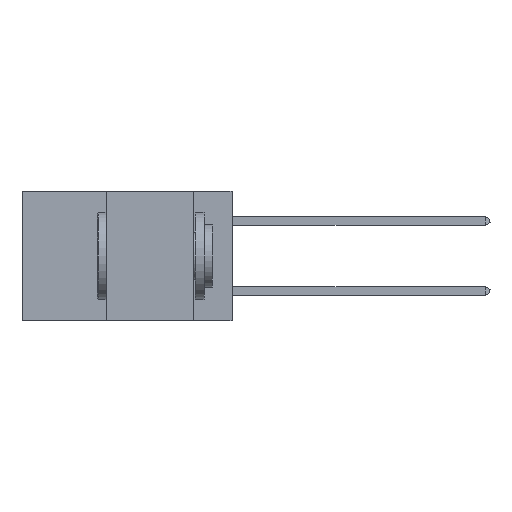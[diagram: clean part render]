
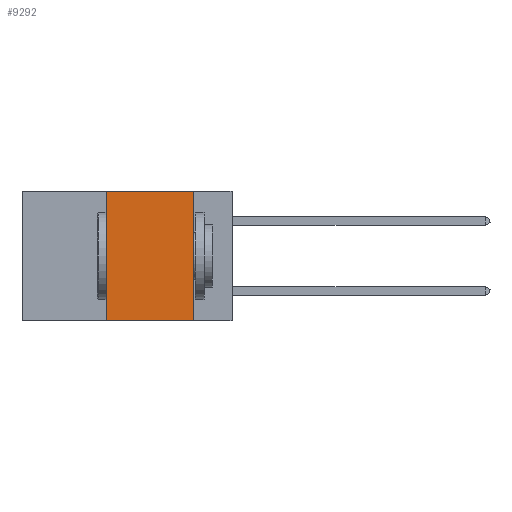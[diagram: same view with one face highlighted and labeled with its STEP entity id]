
A CAD part, left-side view. The second image highlights one B-rep face of the part: STEP entity #9292.
In plain terms, the highlighted planar face has unit normal (-1, 0, 0).
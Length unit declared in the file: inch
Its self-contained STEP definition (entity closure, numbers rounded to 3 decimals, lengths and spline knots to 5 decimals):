
#130 = LINE ( 'NONE', #16089, #18348 ) ;
#188 = CARTESIAN_POINT ( 'NONE',  ( 0., 0.36, -0.37 ) ) ;
#227 = DIRECTION ( 'NONE',  ( 0., -1., 0. ) ) ;
#384 = VERTEX_POINT ( 'NONE', #5617 ) ;
#528 = CARTESIAN_POINT ( 'NONE',  ( 0., 0.6, 0. ) ) ;
#1034 = FACE_OUTER_BOUND ( 'NONE', #13926, .T. ) ;
#1112 = EDGE_CURVE ( 'NONE', #384, #7314, #14309, .T. ) ;
#1474 = CARTESIAN_POINT ( 'NONE',  ( 0., 0.6, -0.37 ) ) ;
#2143 = DIRECTION ( 'NONE',  ( 0., 0., -1. ) ) ;
#2890 = CARTESIAN_POINT ( 'NONE',  ( 0., 0.6, 0. ) ) ;
#3278 = VERTEX_POINT ( 'NONE', #5390 ) ;
#3637 = VERTEX_POINT ( 'NONE', #188 ) ;
#4757 = DIRECTION ( 'NONE',  ( 0., 0., -1. ) ) ;
#5390 = CARTESIAN_POINT ( 'NONE',  ( 0., 0.11, -0.37 ) ) ;
#5617 = CARTESIAN_POINT ( 'NONE',  ( 0., 0.36, 0. ) ) ;
#5799 = VECTOR ( 'NONE', #15838, 39.37008 ) ;
#6198 = VECTOR ( 'NONE', #17693, 39.37008 ) ;
#6420 = ORIENTED_EDGE ( 'NONE', *, *, #6874, .F. ) ;
#6874 = EDGE_CURVE ( 'NONE', #7314, #3278, #130, .T. ) ;
#7314 = VERTEX_POINT ( 'NONE', #18262 ) ;
#7462 = EDGE_CURVE ( 'NONE', #3637, #3278, #9644, .T. ) ;
#7794 = ORIENTED_EDGE ( 'NONE', *, *, #7462, .T. ) ;
#9292 = ADVANCED_FACE ( 'NONE', ( #1034 ), #9435, .F. ) ;
#9362 = CARTESIAN_POINT ( 'NONE',  ( 0., 0.36, 0. ) ) ;
#9435 = PLANE ( 'NONE',  #14314 ) ;
#9585 = LINE ( 'NONE', #9362, #6198 ) ;
#9644 = LINE ( 'NONE', #1474, #5799 ) ;
#10105 = VECTOR ( 'NONE', #227, 39.37008 ) ;
#10860 = DIRECTION ( 'NONE',  ( 1., 0., 0. ) ) ;
#11134 = ORIENTED_EDGE ( 'NONE', *, *, #18006, .F. ) ;
#13926 = EDGE_LOOP ( 'NONE', ( #6420, #17631, #11134, #7794 ) ) ;
#14309 = LINE ( 'NONE', #2890, #10105 ) ;
#14314 = AXIS2_PLACEMENT_3D ( 'NONE', #528, #10860, #2143 ) ;
#15838 = DIRECTION ( 'NONE',  ( 0., -1., 0. ) ) ;
#16089 = CARTESIAN_POINT ( 'NONE',  ( 0., 0.11, 0. ) ) ;
#17631 = ORIENTED_EDGE ( 'NONE', *, *, #1112, .F. ) ;
#17693 = DIRECTION ( 'NONE',  ( 0., 0., 1. ) ) ;
#18006 = EDGE_CURVE ( 'NONE', #3637, #384, #9585, .T. ) ;
#18262 = CARTESIAN_POINT ( 'NONE',  ( 0., 0.11, 0. ) ) ;
#18348 = VECTOR ( 'NONE', #4757, 39.37008 ) ;
